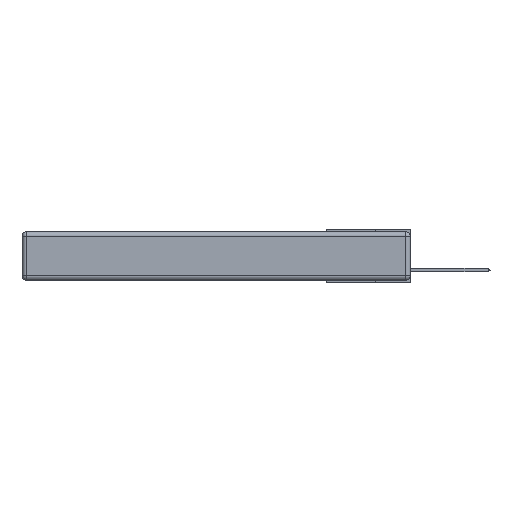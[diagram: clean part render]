
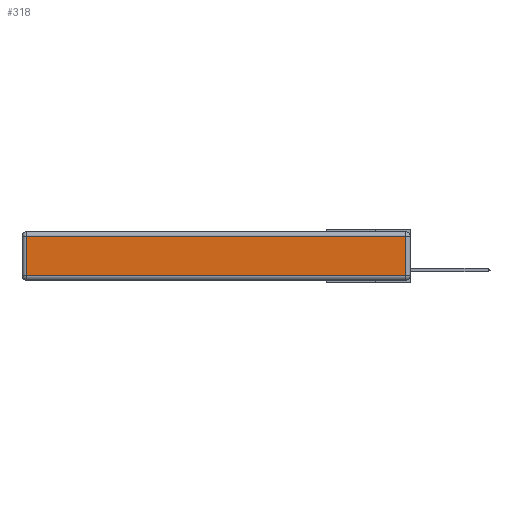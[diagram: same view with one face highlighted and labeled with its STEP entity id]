
A CAD part, left-side view. The second image highlights one B-rep face of the part: STEP entity #318.
In plain terms, the highlighted planar face has unit normal (-1, 0, 0).
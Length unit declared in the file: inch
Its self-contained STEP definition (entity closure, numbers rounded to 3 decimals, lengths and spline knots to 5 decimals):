
#318 = ADVANCED_FACE ( 'NONE', ( #793 ), #12749, .T. ) ;
#508 = DIRECTION ( 'NONE',  ( 0., -1., 0. ) ) ;
#793 = FACE_OUTER_BOUND ( 'NONE', #2346, .T. ) ;
#946 = CARTESIAN_POINT ( 'NONE',  ( 0., 0.03, -0.313 ) ) ;
#992 = ORIENTED_EDGE ( 'NONE', *, *, #2167, .T. ) ;
#1637 = EDGE_CURVE ( 'NONE', #8139, #6343, #8513, .T. ) ;
#1835 = CARTESIAN_POINT ( 'NONE',  ( 0., 2.72, -0.313 ) ) ;
#1846 = DIRECTION ( 'NONE',  ( 0., 1., 0. ) ) ;
#2005 = VERTEX_POINT ( 'NONE', #946 ) ;
#2167 = EDGE_CURVE ( 'NONE', #2005, #5699, #4013, .T. ) ;
#2346 = EDGE_LOOP ( 'NONE', ( #5742, #992, #6282, #8430 ) ) ;
#2571 = CARTESIAN_POINT ( 'NONE',  ( 0., 0.03, -0.343 ) ) ;
#2615 = VECTOR ( 'NONE', #1846, 39.37008 ) ;
#3086 = CARTESIAN_POINT ( 'NONE',  ( 0., 2.75, -0.03 ) ) ;
#3843 = LINE ( 'NONE', #4479, #8542 ) ;
#3974 = DIRECTION ( 'NONE',  ( 0., 0., -1. ) ) ;
#4013 = LINE ( 'NONE', #2571, #8494 ) ;
#4479 = CARTESIAN_POINT ( 'NONE',  ( 0., 0., -0.313 ) ) ;
#4823 = DIRECTION ( 'NONE',  ( -1., 0., 0. ) ) ;
#4833 = CARTESIAN_POINT ( 'NONE',  ( 0., 0.03, -0.03 ) ) ;
#4873 = DIRECTION ( 'NONE',  ( 0., 0., 1. ) ) ;
#4922 = CARTESIAN_POINT ( 'NONE',  ( 0., 0., -0.343 ) ) ;
#5612 = VECTOR ( 'NONE', #3974, 39.37008 ) ;
#5699 = VERTEX_POINT ( 'NONE', #4833 ) ;
#5742 = ORIENTED_EDGE ( 'NONE', *, *, #6208, .T. ) ;
#6208 = EDGE_CURVE ( 'NONE', #6343, #2005, #3843, .T. ) ;
#6282 = ORIENTED_EDGE ( 'NONE', *, *, #16641, .T. ) ;
#6343 = VERTEX_POINT ( 'NONE', #1835 ) ;
#8139 = VERTEX_POINT ( 'NONE', #10033 ) ;
#8330 = LINE ( 'NONE', #3086, #2615 ) ;
#8430 = ORIENTED_EDGE ( 'NONE', *, *, #1637, .T. ) ;
#8494 = VECTOR ( 'NONE', #8895, 39.37008 ) ;
#8513 = LINE ( 'NONE', #14366, #5612 ) ;
#8542 = VECTOR ( 'NONE', #508, 39.37008 ) ;
#8895 = DIRECTION ( 'NONE',  ( 0., 0., 1. ) ) ;
#9689 = AXIS2_PLACEMENT_3D ( 'NONE', #4922, #4823, #4873 ) ;
#10033 = CARTESIAN_POINT ( 'NONE',  ( 0., 2.72, -0.03 ) ) ;
#12749 = PLANE ( 'NONE',  #9689 ) ;
#14366 = CARTESIAN_POINT ( 'NONE',  ( 0., 2.72, -0.343 ) ) ;
#16641 = EDGE_CURVE ( 'NONE', #5699, #8139, #8330, .T. ) ;
